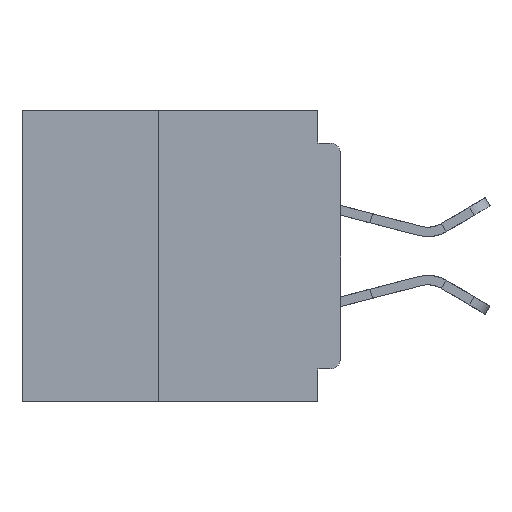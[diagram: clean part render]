
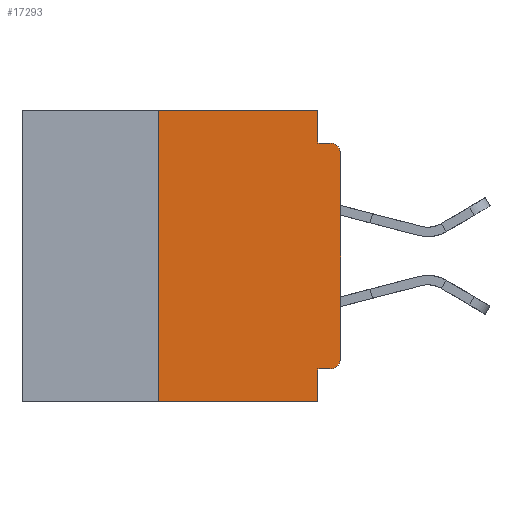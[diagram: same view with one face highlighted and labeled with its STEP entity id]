
A CAD part, left-side view. The second image highlights one B-rep face of the part: STEP entity #17293.
In plain terms, the highlighted planar face has unit normal (-1, 0, 0).
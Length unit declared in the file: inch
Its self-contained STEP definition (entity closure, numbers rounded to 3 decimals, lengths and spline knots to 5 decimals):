
#33 = CARTESIAN_POINT ( 'NONE',  ( 0., 0.031, -0.355 ) ) ;
#183 = ORIENTED_EDGE ( 'NONE', *, *, #32873, .F. ) ;
#493 = EDGE_CURVE ( 'NONE', #1588, #3901, #32712, .T. ) ;
#1588 = VERTEX_POINT ( 'NONE', #37538 ) ;
#2012 = CARTESIAN_POINT ( 'NONE',  ( 0., 0., 0. ) ) ;
#2824 = LINE ( 'NONE', #28226, #9987 ) ;
#3901 = VERTEX_POINT ( 'NONE', #10329 ) ;
#3953 = ORIENTED_EDGE ( 'NONE', *, *, #27186, .F. ) ;
#4033 = CARTESIAN_POINT ( 'NONE',  ( 0., 0.015, -0.045 ) ) ;
#4257 = AXIS2_PLACEMENT_3D ( 'NONE', #27523, #10168, #30392 ) ;
#4305 = LINE ( 'NONE', #27681, #34432 ) ;
#4467 = VECTOR ( 'NONE', #15625, 39.37008 ) ;
#5412 = VECTOR ( 'NONE', #12477, 39.37008 ) ;
#6263 = CARTESIAN_POINT ( 'NONE',  ( 0., 0.031, -0.4 ) ) ;
#7581 = DIRECTION ( 'NONE',  ( 0., 0., -1. ) ) ;
#7733 = AXIS2_PLACEMENT_3D ( 'NONE', #22589, #8064, #28419 ) ;
#8064 = DIRECTION ( 'NONE',  ( 1., 0., 0. ) ) ;
#9076 = VERTEX_POINT ( 'NONE', #21554 ) ;
#9078 = DIRECTION ( 'NONE',  ( 0., 0., 1. ) ) ;
#9474 = DIRECTION ( 'NONE',  ( 0., 0., 1. ) ) ;
#9678 = EDGE_CURVE ( 'NONE', #35585, #14050, #33814, .T. ) ;
#9987 = VECTOR ( 'NONE', #10881, 39.37008 ) ;
#10168 = DIRECTION ( 'NONE',  ( -1., 0., 0. ) ) ;
#10329 = CARTESIAN_POINT ( 'NONE',  ( 0., 0., -0.06 ) ) ;
#10440 = DIRECTION ( 'NONE',  ( 0., -1., 0. ) ) ;
#10775 = VECTOR ( 'NONE', #24073, 39.37008 ) ;
#10867 = EDGE_CURVE ( 'NONE', #30951, #32190, #28799, .T. ) ;
#10881 = DIRECTION ( 'NONE',  ( 0., -1., 0. ) ) ;
#11436 = AXIS2_PLACEMENT_3D ( 'NONE', #30770, #13426, #33659 ) ;
#11509 = VECTOR ( 'NONE', #9474, 39.37008 ) ;
#12374 = EDGE_CURVE ( 'NONE', #35585, #1588, #37099, .T. ) ;
#12476 = ORIENTED_EDGE ( 'NONE', *, *, #12374, .T. ) ;
#12477 = DIRECTION ( 'NONE',  ( 0., -1., 0. ) ) ;
#12492 = LINE ( 'NONE', #27202, #4467 ) ;
#12803 = EDGE_CURVE ( 'NONE', #30951, #9076, #35365, .T. ) ;
#13426 = DIRECTION ( 'NONE',  ( -1., 0., 0. ) ) ;
#13680 = EDGE_CURVE ( 'NONE', #9076, #34150, #4305, .T. ) ;
#14050 = VERTEX_POINT ( 'NONE', #33 ) ;
#14724 = EDGE_CURVE ( 'NONE', #34150, #23567, #25893, .T. ) ;
#14797 = CARTESIAN_POINT ( 'NONE',  ( 0., 0.25, -0.4 ) ) ;
#15547 = ORIENTED_EDGE ( 'NONE', *, *, #9678, .F. ) ;
#15625 = DIRECTION ( 'NONE',  ( 0., 0., -1. ) ) ;
#16557 = ORIENTED_EDGE ( 'NONE', *, *, #33667, .T. ) ;
#17293 = ADVANCED_FACE ( 'NONE', ( #33302 ), #34050, .F. ) ;
#20048 = VECTOR ( 'NONE', #9078, 39.37008 ) ;
#20069 = CIRCLE ( 'NONE', #11436, 0.015 ) ;
#21128 = CARTESIAN_POINT ( 'NONE',  ( 0., 0., -0.355 ) ) ;
#21237 = CARTESIAN_POINT ( 'NONE',  ( 0., 0.25, -0.4 ) ) ;
#21554 = CARTESIAN_POINT ( 'NONE',  ( 0., 0.25, 0. ) ) ;
#22589 = CARTESIAN_POINT ( 'NONE',  ( 0., 0.437, 0. ) ) ;
#22834 = ORIENTED_EDGE ( 'NONE', *, *, #14724, .F. ) ;
#22913 = VERTEX_POINT ( 'NONE', #4033 ) ;
#23567 = VERTEX_POINT ( 'NONE', #29989 ) ;
#24073 = DIRECTION ( 'NONE',  ( 0., 1., 0. ) ) ;
#25893 = LINE ( 'NONE', #27961, #32605 ) ;
#26622 = ORIENTED_EDGE ( 'NONE', *, *, #493, .T. ) ;
#27186 = EDGE_CURVE ( 'NONE', #23567, #22913, #2824, .T. ) ;
#27202 = CARTESIAN_POINT ( 'NONE',  ( 0., 0.031, -0.4 ) ) ;
#27523 = CARTESIAN_POINT ( 'NONE',  ( 0., 0.015, -0.34 ) ) ;
#27681 = CARTESIAN_POINT ( 'NONE',  ( 0., 0.437, 0. ) ) ;
#27961 = CARTESIAN_POINT ( 'NONE',  ( 0., 0.031, 0. ) ) ;
#28226 = CARTESIAN_POINT ( 'NONE',  ( 0., 0., -0.045 ) ) ;
#28419 = DIRECTION ( 'NONE',  ( 0., 0., -1. ) ) ;
#28655 = EDGE_LOOP ( 'NONE', ( #26622, #16557, #3953, #22834, #34089, #33372, #33915, #183, #15547, #12476 ) ) ;
#28799 = LINE ( 'NONE', #29781, #5412 ) ;
#29781 = CARTESIAN_POINT ( 'NONE',  ( 0., 0.437, -0.4 ) ) ;
#29989 = CARTESIAN_POINT ( 'NONE',  ( 0., 0.031, -0.045 ) ) ;
#30392 = DIRECTION ( 'NONE',  ( 0., 0., -1. ) ) ;
#30500 = CARTESIAN_POINT ( 'NONE',  ( 0., 0.031, 0. ) ) ;
#30770 = CARTESIAN_POINT ( 'NONE',  ( 0., 0.015, -0.06 ) ) ;
#30951 = VERTEX_POINT ( 'NONE', #21237 ) ;
#32190 = VERTEX_POINT ( 'NONE', #6263 ) ;
#32605 = VECTOR ( 'NONE', #7581, 39.37008 ) ;
#32712 = LINE ( 'NONE', #2012, #11509 ) ;
#32873 = EDGE_CURVE ( 'NONE', #14050, #32190, #12492, .T. ) ;
#33302 = FACE_OUTER_BOUND ( 'NONE', #28655, .T. ) ;
#33372 = ORIENTED_EDGE ( 'NONE', *, *, #12803, .F. ) ;
#33659 = DIRECTION ( 'NONE',  ( 0., 0., -1. ) ) ;
#33667 = EDGE_CURVE ( 'NONE', #3901, #22913, #20069, .T. ) ;
#33814 = LINE ( 'NONE', #21128, #10775 ) ;
#33915 = ORIENTED_EDGE ( 'NONE', *, *, #10867, .T. ) ;
#34050 = PLANE ( 'NONE',  #7733 ) ;
#34089 = ORIENTED_EDGE ( 'NONE', *, *, #13680, .F. ) ;
#34150 = VERTEX_POINT ( 'NONE', #30500 ) ;
#34432 = VECTOR ( 'NONE', #10440, 39.37008 ) ;
#35365 = LINE ( 'NONE', #14797, #20048 ) ;
#35585 = VERTEX_POINT ( 'NONE', #36945 ) ;
#36945 = CARTESIAN_POINT ( 'NONE',  ( 0., 0.015, -0.355 ) ) ;
#37099 = CIRCLE ( 'NONE', #4257, 0.015 ) ;
#37538 = CARTESIAN_POINT ( 'NONE',  ( 0., 0., -0.34 ) ) ;
